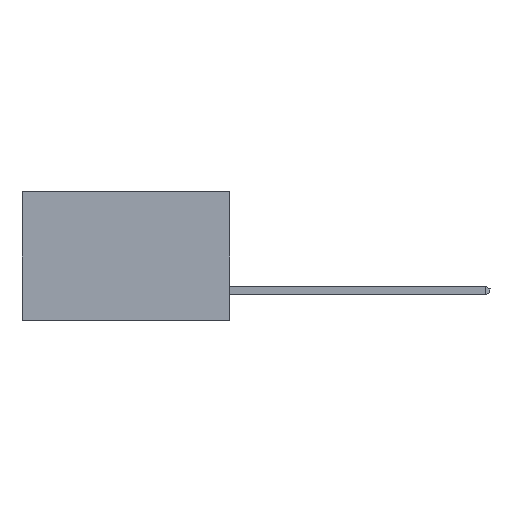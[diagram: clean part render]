
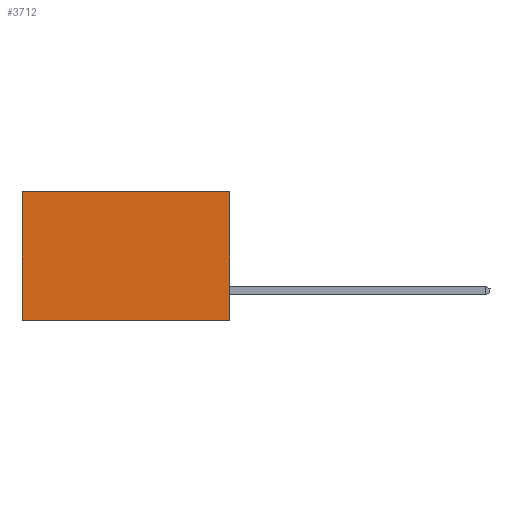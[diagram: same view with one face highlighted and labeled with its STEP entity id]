
A CAD part, left-side view. The second image highlights one B-rep face of the part: STEP entity #3712.
In plain terms, the highlighted planar face has unit normal (-1, 0, 0).
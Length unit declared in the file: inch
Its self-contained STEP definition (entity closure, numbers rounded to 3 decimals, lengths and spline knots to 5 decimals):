
#1312 = CARTESIAN_POINT ( 'NONE',  ( 0.2615, 0.6, 0. ) ) ;
#1990 = CARTESIAN_POINT ( 'NONE',  ( 0.2615, 0., 0. ) ) ;
#2061 = ORIENTED_EDGE ( 'NONE', *, *, #4370, .F. ) ;
#3712 = ADVANCED_FACE ( 'NONE', ( #6221 ), #14679, .F. ) ;
#4340 = VERTEX_POINT ( 'NONE', #6133 ) ;
#4370 = EDGE_CURVE ( 'NONE', #4340, #15788, #17952, .T. ) ;
#5258 = LINE ( 'NONE', #1990, #12733 ) ;
#6133 = CARTESIAN_POINT ( 'NONE',  ( 0.2615, 0., 0. ) ) ;
#6221 = FACE_OUTER_BOUND ( 'NONE', #18104, .T. ) ;
#6278 = CARTESIAN_POINT ( 'NONE',  ( 0.2615, 0.6, -0.37 ) ) ;
#6325 = DIRECTION ( 'NONE',  ( 0., 0., -1. ) ) ;
#6535 = DIRECTION ( 'NONE',  ( 1., 0., 0. ) ) ;
#6662 = ORIENTED_EDGE ( 'NONE', *, *, #10678, .T. ) ;
#6932 = CARTESIAN_POINT ( 'NONE',  ( 0.2615, 0., -0.37 ) ) ;
#7134 = ORIENTED_EDGE ( 'NONE', *, *, #19628, .F. ) ;
#7746 = EDGE_CURVE ( 'NONE', #4340, #16948, #5258, .T. ) ;
#8340 = DIRECTION ( 'NONE',  ( 0., 1., 0. ) ) ;
#8357 = VERTEX_POINT ( 'NONE', #10960 ) ;
#8916 = CARTESIAN_POINT ( 'NONE',  ( 0.2615, 0., -0.37 ) ) ;
#9684 = CARTESIAN_POINT ( 'NONE',  ( 0.2615, 0., -0.37 ) ) ;
#9769 = CARTESIAN_POINT ( 'NONE',  ( 0.2615, 0., -0.37 ) ) ;
#10678 = EDGE_CURVE ( 'NONE', #16948, #8357, #21266, .T. ) ;
#10960 = CARTESIAN_POINT ( 'NONE',  ( 0.2615, 0.6, -0.37 ) ) ;
#12478 = VECTOR ( 'NONE', #21366, 39.37008 ) ;
#12733 = VECTOR ( 'NONE', #8340, 39.37008 ) ;
#13430 = LINE ( 'NONE', #6932, #13564 ) ;
#13564 = VECTOR ( 'NONE', #19934, 39.37008 ) ;
#14679 = PLANE ( 'NONE',  #20778 ) ;
#15788 = VERTEX_POINT ( 'NONE', #8916 ) ;
#16948 = VERTEX_POINT ( 'NONE', #1312 ) ;
#17314 = ORIENTED_EDGE ( 'NONE', *, *, #7746, .T. ) ;
#17952 = LINE ( 'NONE', #9684, #20182 ) ;
#18104 = EDGE_LOOP ( 'NONE', ( #6662, #7134, #2061, #17314 ) ) ;
#19270 = DIRECTION ( 'NONE',  ( 0., 0., -1. ) ) ;
#19628 = EDGE_CURVE ( 'NONE', #15788, #8357, #13430, .T. ) ;
#19934 = DIRECTION ( 'NONE',  ( 0., 1., 0. ) ) ;
#20182 = VECTOR ( 'NONE', #19270, 39.37008 ) ;
#20778 = AXIS2_PLACEMENT_3D ( 'NONE', #9769, #6535, #6325 ) ;
#21266 = LINE ( 'NONE', #6278, #12478 ) ;
#21366 = DIRECTION ( 'NONE',  ( 0., 0., -1. ) ) ;
